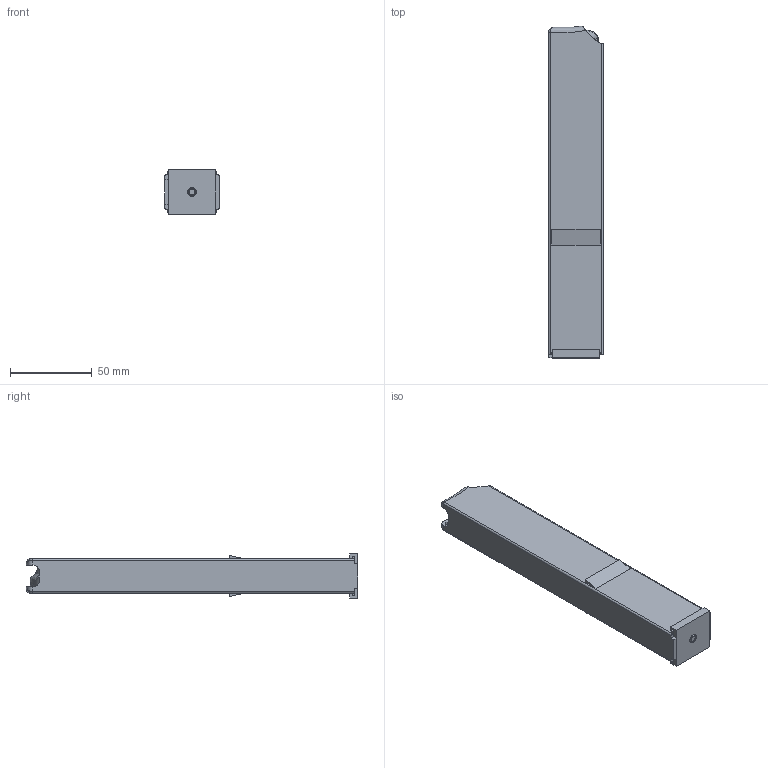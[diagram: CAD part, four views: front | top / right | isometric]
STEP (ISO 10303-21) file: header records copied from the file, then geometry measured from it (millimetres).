
FILE_DESCRIPTION (( 'STEP AP214' ), '1' );
FILE_NAME ('uzi_mag_assem.STEP', '2013-06-02T20:15:40', ( '' ), ( '' ), 'SwSTEP 2.0', 'SolidWorks 2013', '' );
FILE_SCHEMA (( 'AUTOMOTIVE_DESIGN' ));
Length unit declared in the file: millimetre
Products named in the file (5): lock_plate; mag_body; follower; floorplate; uzi_mag_assem
Assembly tree (4 placements, depth 2):
  uzi_mag_assem
    floorplate
    follower
    mag_body
    lock_plate
Bounding box: 33.5 x 202.81 x 27 mm (x, y, z)
Volume: 49004.5 mm3; surface area: 46755.7 mm2
Topology: 4 solids, 4 shells, 271 faces, 722 edges, 469 vertices
Faces by surface type: plane 135, bspline 85, cylinder 39, sphere 6, torus 6
Entity records: 14243 total; most frequent: CARTESIAN_POINT 7881, ORIENTED_EDGE 1432, DIRECTION 998, EDGE_CURVE 716, VERTEX_POINT 467, LINE 446, VECTOR 446, EDGE_LOOP 301
